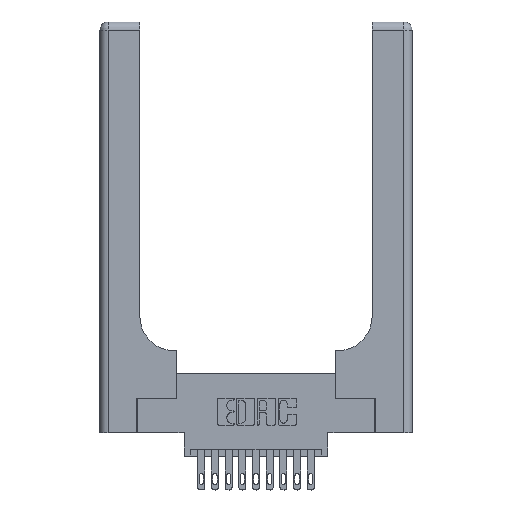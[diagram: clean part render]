
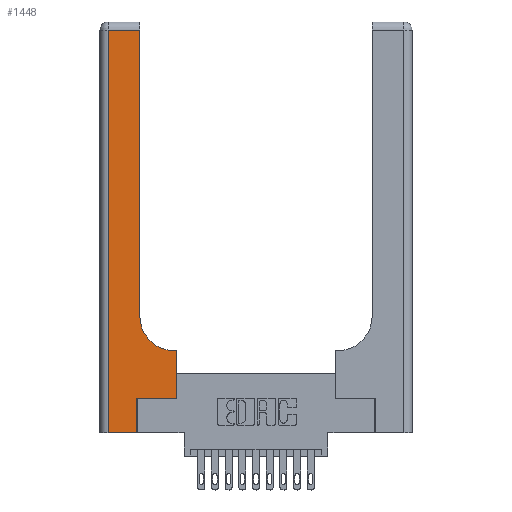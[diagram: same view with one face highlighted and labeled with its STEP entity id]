
A CAD part, top view. The second image highlights one B-rep face of the part: STEP entity #1448.
In plain terms, the highlighted planar face has unit normal (0, 0, 1).
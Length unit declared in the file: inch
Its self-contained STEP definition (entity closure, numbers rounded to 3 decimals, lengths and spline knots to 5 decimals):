
#157 = EDGE_CURVE ( 'NONE', #4485, #11594, #16522, .T. ) ;
#515 = VERTEX_POINT ( 'NONE', #16772 ) ;
#673 = EDGE_CURVE ( 'NONE', #1157, #16729, #4306, .T. ) ;
#888 = CARTESIAN_POINT ( 'NONE',  ( 0., 2.94, 0.37 ) ) ;
#1148 = VECTOR ( 'NONE', #6419, 39.37008 ) ;
#1157 = VERTEX_POINT ( 'NONE', #8742 ) ;
#1188 = DIRECTION ( 'NONE',  ( 1., 0., 0. ) ) ;
#1291 = EDGE_CURVE ( 'NONE', #7851, #4485, #5310, .T. ) ;
#1448 = ADVANCED_FACE ( 'NONE', ( #7969 ), #7033, .F. ) ;
#1677 = VECTOR ( 'NONE', #4421, 39.37008 ) ;
#1766 = VERTEX_POINT ( 'NONE', #5035 ) ;
#2397 = CIRCLE ( 'NONE', #13192, 0.25 ) ;
#2676 = LINE ( 'NONE', #5555, #1677 ) ;
#2819 = EDGE_CURVE ( 'NONE', #3630, #1766, #12304, .T. ) ;
#3456 = LINE ( 'NONE', #888, #9953 ) ;
#3630 = VERTEX_POINT ( 'NONE', #9494 ) ;
#4306 = LINE ( 'NONE', #10253, #16732 ) ;
#4421 = DIRECTION ( 'NONE',  ( 0., 1., 0. ) ) ;
#4485 = VERTEX_POINT ( 'NONE', #9636 ) ;
#4669 = LINE ( 'NONE', #14206, #6700 ) ;
#5035 = CARTESIAN_POINT ( 'NONE',  ( 0.06, 0., 0.37 ) ) ;
#5037 = EDGE_CURVE ( 'NONE', #515, #12753, #13029, .T. ) ;
#5113 = VECTOR ( 'NONE', #7355, 39.37008 ) ;
#5174 = DIRECTION ( 'NONE',  ( 0., 0., -1. ) ) ;
#5310 = LINE ( 'NONE', #7161, #10193 ) ;
#5555 = CARTESIAN_POINT ( 'NONE',  ( 0.5585, 0.25, 0.37 ) ) ;
#5736 = EDGE_CURVE ( 'NONE', #1766, #7851, #4669, .T. ) ;
#6207 = EDGE_CURVE ( 'NONE', #12753, #3630, #3456, .T. ) ;
#6419 = DIRECTION ( 'NONE',  ( 0., -1., 0. ) ) ;
#6700 = VECTOR ( 'NONE', #15576, 39.37008 ) ;
#7033 = PLANE ( 'NONE',  #13360 ) ;
#7161 = CARTESIAN_POINT ( 'NONE',  ( 0.269, 0., 0.37 ) ) ;
#7355 = DIRECTION ( 'NONE',  ( 0., 1., 0. ) ) ;
#7534 = EDGE_CURVE ( 'NONE', #16729, #515, #2397, .T. ) ;
#7817 = CARTESIAN_POINT ( 'NONE',  ( 0.5415, 0.85, 0.37 ) ) ;
#7851 = VERTEX_POINT ( 'NONE', #10966 ) ;
#7969 = FACE_OUTER_BOUND ( 'NONE', #13313, .T. ) ;
#8167 = VECTOR ( 'NONE', #1188, 39.37008 ) ;
#8572 = ORIENTED_EDGE ( 'NONE', *, *, #7534, .T. ) ;
#8663 = ORIENTED_EDGE ( 'NONE', *, *, #15776, .T. ) ;
#8742 = CARTESIAN_POINT ( 'NONE',  ( 0.5585, 0.6, 0.37 ) ) ;
#8936 = DIRECTION ( 'NONE',  ( 0., 1., 0. ) ) ;
#8939 = CARTESIAN_POINT ( 'NONE',  ( 0.269, 0.25, 0.37 ) ) ;
#9002 = DIRECTION ( 'NONE',  ( -1., 0., 0. ) ) ;
#9148 = CARTESIAN_POINT ( 'NONE',  ( 0.5585, 0.25, 0.37 ) ) ;
#9494 = CARTESIAN_POINT ( 'NONE',  ( 0.06, 2.94, 0.37 ) ) ;
#9605 = ORIENTED_EDGE ( 'NONE', *, *, #673, .T. ) ;
#9636 = CARTESIAN_POINT ( 'NONE',  ( 0.269, 0.25, 0.37 ) ) ;
#9876 = DIRECTION ( 'NONE',  ( -1., 0., 0. ) ) ;
#9953 = VECTOR ( 'NONE', #9876, 39.37008 ) ;
#10193 = VECTOR ( 'NONE', #8936, 39.37008 ) ;
#10218 = CARTESIAN_POINT ( 'NONE',  ( 0.06, 3., 0.37 ) ) ;
#10253 = CARTESIAN_POINT ( 'NONE',  ( 0.2915, 0.6, 0.37 ) ) ;
#10293 = DIRECTION ( 'NONE',  ( 1., 0., 0. ) ) ;
#10966 = CARTESIAN_POINT ( 'NONE',  ( 0.269, 0., 0.37 ) ) ;
#11594 = VERTEX_POINT ( 'NONE', #9148 ) ;
#11676 = ORIENTED_EDGE ( 'NONE', *, *, #2819, .T. ) ;
#11895 = ORIENTED_EDGE ( 'NONE', *, *, #5736, .T. ) ;
#12304 = LINE ( 'NONE', #10218, #1148 ) ;
#12387 = ORIENTED_EDGE ( 'NONE', *, *, #157, .T. ) ;
#12753 = VERTEX_POINT ( 'NONE', #14051 ) ;
#13029 = LINE ( 'NONE', #13723, #5113 ) ;
#13192 = AXIS2_PLACEMENT_3D ( 'NONE', #7817, #5174, #10293 ) ;
#13313 = EDGE_LOOP ( 'NONE', ( #14775, #14857, #11676, #11895, #14688, #12387, #8663, #9605, #8572 ) ) ;
#13360 = AXIS2_PLACEMENT_3D ( 'NONE', #13397, #13505, #16124 ) ;
#13397 = CARTESIAN_POINT ( 'NONE',  ( 0., 3., 0.37 ) ) ;
#13505 = DIRECTION ( 'NONE',  ( 0., 0., -1. ) ) ;
#13535 = CARTESIAN_POINT ( 'NONE',  ( 0.5415, 0.6, 0.37 ) ) ;
#13723 = CARTESIAN_POINT ( 'NONE',  ( 0.2915, 3., 0.37 ) ) ;
#14051 = CARTESIAN_POINT ( 'NONE',  ( 0.2915, 2.94, 0.37 ) ) ;
#14206 = CARTESIAN_POINT ( 'NONE',  ( 0., 0., 0.37 ) ) ;
#14688 = ORIENTED_EDGE ( 'NONE', *, *, #1291, .T. ) ;
#14775 = ORIENTED_EDGE ( 'NONE', *, *, #5037, .T. ) ;
#14857 = ORIENTED_EDGE ( 'NONE', *, *, #6207, .T. ) ;
#15576 = DIRECTION ( 'NONE',  ( 1., 0., 0. ) ) ;
#15776 = EDGE_CURVE ( 'NONE', #11594, #1157, #2676, .T. ) ;
#16124 = DIRECTION ( 'NONE',  ( -1., 0., 0. ) ) ;
#16522 = LINE ( 'NONE', #8939, #8167 ) ;
#16729 = VERTEX_POINT ( 'NONE', #13535 ) ;
#16732 = VECTOR ( 'NONE', #9002, 39.37008 ) ;
#16772 = CARTESIAN_POINT ( 'NONE',  ( 0.2915, 0.85, 0.37 ) ) ;
